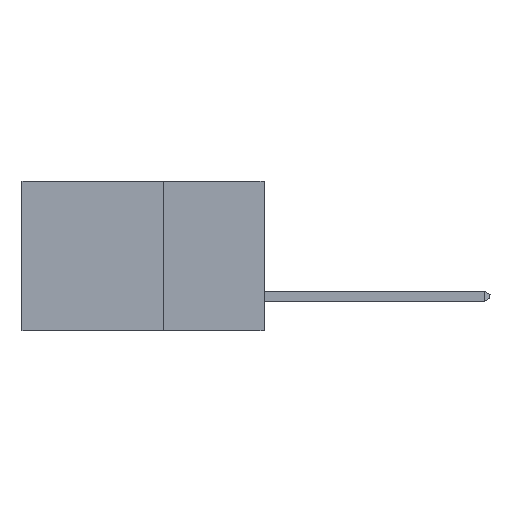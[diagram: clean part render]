
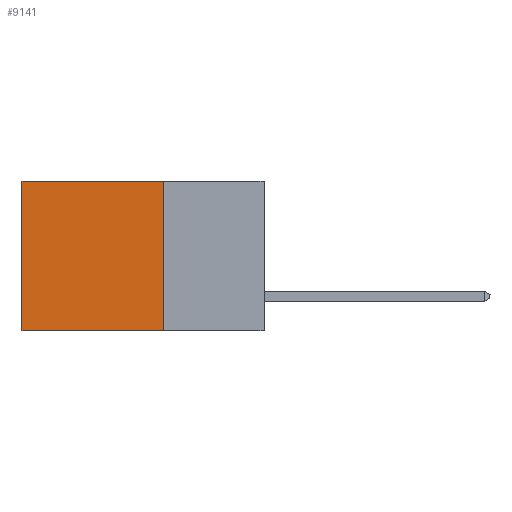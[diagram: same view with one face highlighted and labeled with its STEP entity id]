
A CAD part, left-side view. The second image highlights one B-rep face of the part: STEP entity #9141.
In plain terms, the highlighted planar face has unit normal (-1, 0, 0).
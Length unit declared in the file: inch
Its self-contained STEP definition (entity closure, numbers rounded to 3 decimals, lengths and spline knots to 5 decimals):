
#671 = FACE_OUTER_BOUND ( 'NONE', #9389, .T. ) ;
#680 = EDGE_CURVE ( 'NONE', #7233, #7891, #7439, .T. ) ;
#700 = LINE ( 'NONE', #4600, #4545 ) ;
#743 = ORIENTED_EDGE ( 'NONE', *, *, #6274, .T. ) ;
#1421 = VECTOR ( 'NONE', #7807, 39.37008 ) ;
#1616 = AXIS2_PLACEMENT_3D ( 'NONE', #10164, #1763, #7777 ) ;
#1763 = DIRECTION ( 'NONE',  ( 1., 0., 0. ) ) ;
#2106 = DIRECTION ( 'NONE',  ( 0., 1., 0. ) ) ;
#2442 = EDGE_CURVE ( 'NONE', #10389, #7891, #700, .T. ) ;
#2881 = VECTOR ( 'NONE', #9276, 39.37008 ) ;
#3169 = LINE ( 'NONE', #7841, #1421 ) ;
#4310 = VERTEX_POINT ( 'NONE', #4577 ) ;
#4545 = VECTOR ( 'NONE', #2106, 39.37008 ) ;
#4577 = CARTESIAN_POINT ( 'NONE',  ( 0.298, 0.25, 0. ) ) ;
#4600 = CARTESIAN_POINT ( 'NONE',  ( 0.298, 0.25, -0.37 ) ) ;
#4810 = CARTESIAN_POINT ( 'NONE',  ( 0.298, 0.25, 0. ) ) ;
#5882 = VECTOR ( 'NONE', #5929, 39.37008 ) ;
#5897 = ORIENTED_EDGE ( 'NONE', *, *, #7596, .F. ) ;
#5929 = DIRECTION ( 'NONE',  ( 0., 1., 0. ) ) ;
#6274 = EDGE_CURVE ( 'NONE', #4310, #7233, #6541, .T. ) ;
#6469 = CARTESIAN_POINT ( 'NONE',  ( 0.298, 0.6, 0. ) ) ;
#6541 = LINE ( 'NONE', #4810, #5882 ) ;
#6700 = CARTESIAN_POINT ( 'NONE',  ( 0.298, 0.25, -0.37 ) ) ;
#7233 = VERTEX_POINT ( 'NONE', #6469 ) ;
#7304 = ORIENTED_EDGE ( 'NONE', *, *, #680, .T. ) ;
#7439 = LINE ( 'NONE', #10252, #2881 ) ;
#7596 = EDGE_CURVE ( 'NONE', #4310, #10389, #3169, .T. ) ;
#7777 = DIRECTION ( 'NONE',  ( 0., 0., -1. ) ) ;
#7807 = DIRECTION ( 'NONE',  ( 0., 0., -1. ) ) ;
#7841 = CARTESIAN_POINT ( 'NONE',  ( 0.298, 0.25, 0. ) ) ;
#7891 = VERTEX_POINT ( 'NONE', #10643 ) ;
#7977 = ORIENTED_EDGE ( 'NONE', *, *, #2442, .F. ) ;
#9141 = ADVANCED_FACE ( 'NONE', ( #671 ), #10954, .F. ) ;
#9276 = DIRECTION ( 'NONE',  ( 0., 0., -1. ) ) ;
#9389 = EDGE_LOOP ( 'NONE', ( #7304, #7977, #5897, #743 ) ) ;
#10164 = CARTESIAN_POINT ( 'NONE',  ( 0.298, 0.25, 0. ) ) ;
#10252 = CARTESIAN_POINT ( 'NONE',  ( 0.298, 0.6, 0. ) ) ;
#10389 = VERTEX_POINT ( 'NONE', #6700 ) ;
#10643 = CARTESIAN_POINT ( 'NONE',  ( 0.298, 0.6, -0.37 ) ) ;
#10954 = PLANE ( 'NONE',  #1616 ) ;
